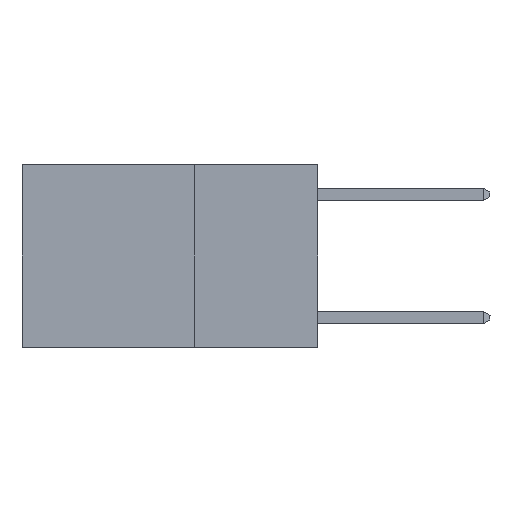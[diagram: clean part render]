
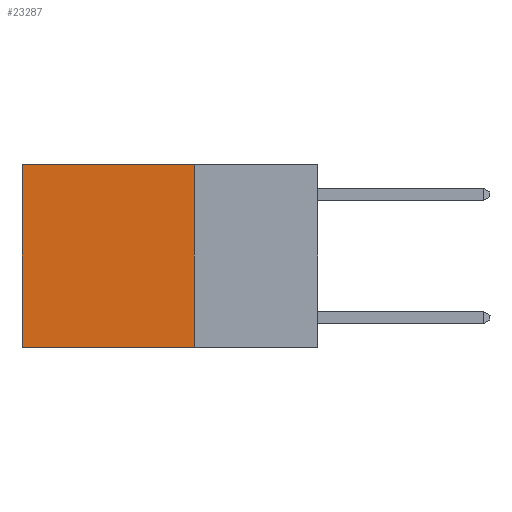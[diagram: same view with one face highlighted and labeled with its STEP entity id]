
A CAD part, left-side view. The second image highlights one B-rep face of the part: STEP entity #23287.
In plain terms, the highlighted planar face has unit normal (-1, 0, 0).
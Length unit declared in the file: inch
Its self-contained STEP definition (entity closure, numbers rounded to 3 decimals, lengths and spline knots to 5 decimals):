
#1294 = VERTEX_POINT ( 'NONE', #6129 ) ;
#1829 = DIRECTION ( 'NONE',  ( 0., 0., -1. ) ) ;
#2262 = EDGE_CURVE ( 'NONE', #1294, #20546, #2482, .T. ) ;
#2482 = LINE ( 'NONE', #10310, #13633 ) ;
#4470 = VERTEX_POINT ( 'NONE', #7616 ) ;
#4765 = LINE ( 'NONE', #30553, #23373 ) ;
#5713 = EDGE_LOOP ( 'NONE', ( #27769, #30806, #22375, #24750 ) ) ;
#5793 = EDGE_CURVE ( 'NONE', #23249, #4470, #23801, .T. ) ;
#6129 = CARTESIAN_POINT ( 'NONE',  ( 0.2625, 0.25, -0.37 ) ) ;
#6732 = VECTOR ( 'NONE', #32099, 39.37008 ) ;
#7616 = CARTESIAN_POINT ( 'NONE',  ( 0.2625, 0.6, 0. ) ) ;
#8250 = EDGE_CURVE ( 'NONE', #4470, #20546, #4765, .T. ) ;
#8257 = DIRECTION ( 'NONE',  ( 0., 0., -1. ) ) ;
#10310 = CARTESIAN_POINT ( 'NONE',  ( 0.2625, 0.25, -0.37 ) ) ;
#11480 = CARTESIAN_POINT ( 'NONE',  ( 0.2625, 0.6, -0.37 ) ) ;
#12912 = CARTESIAN_POINT ( 'NONE',  ( 0.2625, 0.25, 0. ) ) ;
#13012 = CARTESIAN_POINT ( 'NONE',  ( 0.2625, 0.25, 0. ) ) ;
#13633 = VECTOR ( 'NONE', #15621, 39.37008 ) ;
#14675 = EDGE_CURVE ( 'NONE', #23249, #1294, #30268, .T. ) ;
#15621 = DIRECTION ( 'NONE',  ( 0., 1., 0. ) ) ;
#15657 = DIRECTION ( 'NONE',  ( 0., 0., -1. ) ) ;
#15829 = FACE_OUTER_BOUND ( 'NONE', #5713, .T. ) ;
#18896 = CARTESIAN_POINT ( 'NONE',  ( 0.2625, 0.25, 0. ) ) ;
#20299 = AXIS2_PLACEMENT_3D ( 'NONE', #13012, #25760, #15657 ) ;
#20546 = VERTEX_POINT ( 'NONE', #11480 ) ;
#22375 = ORIENTED_EDGE ( 'NONE', *, *, #14675, .F. ) ;
#22702 = VECTOR ( 'NONE', #8257, 39.37008 ) ;
#23249 = VERTEX_POINT ( 'NONE', #12912 ) ;
#23287 = ADVANCED_FACE ( 'NONE', ( #15829 ), #25971, .F. ) ;
#23373 = VECTOR ( 'NONE', #1829, 39.37008 ) ;
#23801 = LINE ( 'NONE', #27136, #6732 ) ;
#24750 = ORIENTED_EDGE ( 'NONE', *, *, #5793, .T. ) ;
#25760 = DIRECTION ( 'NONE',  ( 1., 0., 0. ) ) ;
#25971 = PLANE ( 'NONE',  #20299 ) ;
#27136 = CARTESIAN_POINT ( 'NONE',  ( 0.2625, 0.25, 0. ) ) ;
#27769 = ORIENTED_EDGE ( 'NONE', *, *, #8250, .T. ) ;
#30268 = LINE ( 'NONE', #18896, #22702 ) ;
#30553 = CARTESIAN_POINT ( 'NONE',  ( 0.2625, 0.6, 0. ) ) ;
#30806 = ORIENTED_EDGE ( 'NONE', *, *, #2262, .F. ) ;
#32099 = DIRECTION ( 'NONE',  ( 0., 1., 0. ) ) ;
